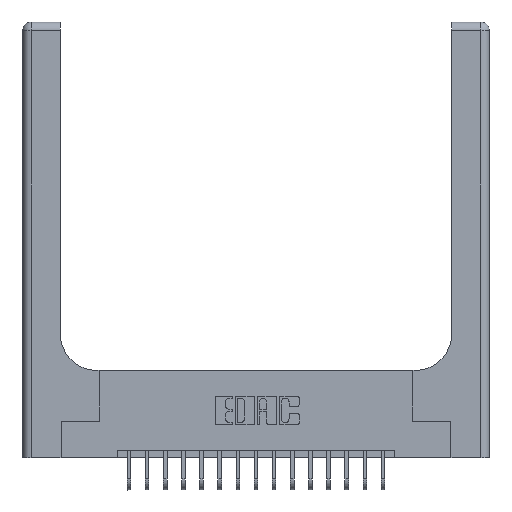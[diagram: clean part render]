
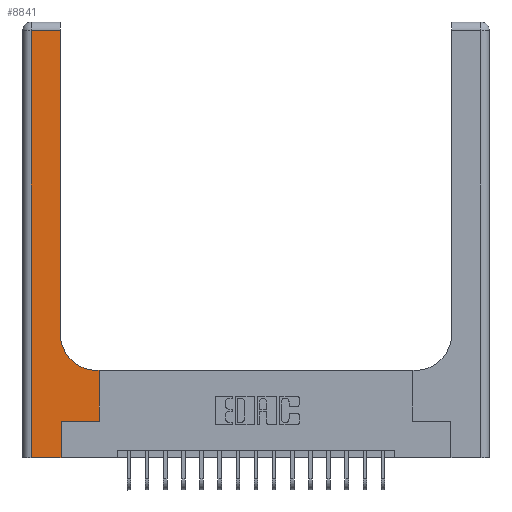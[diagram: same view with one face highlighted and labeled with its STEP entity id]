
A CAD part, top view. The second image highlights one B-rep face of the part: STEP entity #8841.
In plain terms, the highlighted planar face has unit normal (0, 0, 1).
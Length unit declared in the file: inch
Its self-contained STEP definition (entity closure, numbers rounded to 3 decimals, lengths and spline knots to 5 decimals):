
#110 = EDGE_CURVE ( 'NONE', #10247, #282, #4777, .T. ) ;
#227 = CARTESIAN_POINT ( 'NONE',  ( 0.26, 2.94, 0.37 ) ) ;
#282 = VERTEX_POINT ( 'NONE', #8827 ) ;
#332 = LINE ( 'NONE', #10651, #8175 ) ;
#1098 = VECTOR ( 'NONE', #10964, 39.37008 ) ;
#1131 = LINE ( 'NONE', #14423, #17380 ) ;
#1418 = DIRECTION ( 'NONE',  ( 0., 0., -1. ) ) ;
#1751 = DIRECTION ( 'NONE',  ( 0., 0., -1. ) ) ;
#2239 = DIRECTION ( 'NONE',  ( 0., 1., 0. ) ) ;
#2355 = LINE ( 'NONE', #10632, #17366 ) ;
#2410 = EDGE_CURVE ( 'NONE', #8471, #15333, #11930, .T. ) ;
#3221 = EDGE_CURVE ( 'NONE', #282, #6428, #16419, .T. ) ;
#3464 = DIRECTION ( 'NONE',  ( 0., 1., 0. ) ) ;
#3870 = EDGE_CURVE ( 'NONE', #9569, #4636, #1131, .T. ) ;
#4448 = EDGE_LOOP ( 'NONE', ( #10275, #13189, #12014, #18849, #20106, #5891, #11778, #18100, #5657 ) ) ;
#4636 = VERTEX_POINT ( 'NONE', #15033 ) ;
#4660 = CARTESIAN_POINT ( 'NONE',  ( 0., 2.94, 0.37 ) ) ;
#4743 = DIRECTION ( 'NONE',  ( 0., 1., 0. ) ) ;
#4777 = LINE ( 'NONE', #7968, #1098 ) ;
#4818 = VERTEX_POINT ( 'NONE', #17353 ) ;
#5657 = ORIENTED_EDGE ( 'NONE', *, *, #3221, .T. ) ;
#5891 = ORIENTED_EDGE ( 'NONE', *, *, #7492, .T. ) ;
#6418 = CARTESIAN_POINT ( 'NONE',  ( 0.265, 0., 0.37 ) ) ;
#6428 = VERTEX_POINT ( 'NONE', #19565 ) ;
#6442 = EDGE_CURVE ( 'NONE', #14029, #10247, #332, .T. ) ;
#6672 = VECTOR ( 'NONE', #13729, 39.37008 ) ;
#7492 = EDGE_CURVE ( 'NONE', #4636, #14029, #11863, .T. ) ;
#7692 = VECTOR ( 'NONE', #4743, 39.37008 ) ;
#7725 = CARTESIAN_POINT ( 'NONE',  ( 0.51, 0.85, 0.37 ) ) ;
#7849 = DIRECTION ( 'NONE',  ( 1., 0., 0. ) ) ;
#7946 = VECTOR ( 'NONE', #12591, 39.37008 ) ;
#7968 = CARTESIAN_POINT ( 'NONE',  ( 0.26, 0.6, 0.37 ) ) ;
#7972 = CARTESIAN_POINT ( 'NONE',  ( 0.528, 0.6, 0.37 ) ) ;
#8175 = VECTOR ( 'NONE', #2239, 39.37008 ) ;
#8471 = VERTEX_POINT ( 'NONE', #227 ) ;
#8827 = CARTESIAN_POINT ( 'NONE',  ( 0.51, 0.6, 0.37 ) ) ;
#8841 = ADVANCED_FACE ( 'NONE', ( #13992 ), #14141, .F. ) ;
#9569 = VERTEX_POINT ( 'NONE', #6418 ) ;
#9953 = DIRECTION ( 'NONE',  ( -1., 0., 0. ) ) ;
#10247 = VERTEX_POINT ( 'NONE', #7972 ) ;
#10275 = ORIENTED_EDGE ( 'NONE', *, *, #15629, .T. ) ;
#10495 = CARTESIAN_POINT ( 'NONE',  ( 0., 0., 0.37 ) ) ;
#10632 = CARTESIAN_POINT ( 'NONE',  ( 0.06, 3., 0.37 ) ) ;
#10651 = CARTESIAN_POINT ( 'NONE',  ( 0.528, 0.25, 0.37 ) ) ;
#10964 = DIRECTION ( 'NONE',  ( -1., 0., 0. ) ) ;
#11034 = CARTESIAN_POINT ( 'NONE',  ( 0.26, 3., 0.37 ) ) ;
#11778 = ORIENTED_EDGE ( 'NONE', *, *, #6442, .T. ) ;
#11863 = LINE ( 'NONE', #18374, #6672 ) ;
#11930 = LINE ( 'NONE', #4660, #7946 ) ;
#12014 = ORIENTED_EDGE ( 'NONE', *, *, #13231, .T. ) ;
#12591 = DIRECTION ( 'NONE',  ( -1., 0., 0. ) ) ;
#12728 = DIRECTION ( 'NONE',  ( 0., -1., 0. ) ) ;
#12943 = CARTESIAN_POINT ( 'NONE',  ( 0.528, 0.25, 0.37 ) ) ;
#13189 = ORIENTED_EDGE ( 'NONE', *, *, #2410, .T. ) ;
#13231 = EDGE_CURVE ( 'NONE', #15333, #4818, #2355, .T. ) ;
#13729 = DIRECTION ( 'NONE',  ( 1., 0., 0. ) ) ;
#13992 = FACE_OUTER_BOUND ( 'NONE', #4448, .T. ) ;
#14029 = VERTEX_POINT ( 'NONE', #12943 ) ;
#14070 = AXIS2_PLACEMENT_3D ( 'NONE', #7725, #1418, #7849 ) ;
#14141 = PLANE ( 'NONE',  #14687 ) ;
#14423 = CARTESIAN_POINT ( 'NONE',  ( 0.265, 0., 0.37 ) ) ;
#14687 = AXIS2_PLACEMENT_3D ( 'NONE', #17601, #1751, #9953 ) ;
#14967 = CARTESIAN_POINT ( 'NONE',  ( 0.06, 2.94, 0.37 ) ) ;
#15033 = CARTESIAN_POINT ( 'NONE',  ( 0.265, 0.25, 0.37 ) ) ;
#15333 = VERTEX_POINT ( 'NONE', #14967 ) ;
#15421 = DIRECTION ( 'NONE',  ( 1., 0., 0. ) ) ;
#15596 = LINE ( 'NONE', #11034, #7692 ) ;
#15629 = EDGE_CURVE ( 'NONE', #6428, #8471, #15596, .T. ) ;
#15730 = LINE ( 'NONE', #10495, #19957 ) ;
#16419 = CIRCLE ( 'NONE', #14070, 0.25 ) ;
#17353 = CARTESIAN_POINT ( 'NONE',  ( 0.06, 0., 0.37 ) ) ;
#17366 = VECTOR ( 'NONE', #12728, 39.37008 ) ;
#17380 = VECTOR ( 'NONE', #3464, 39.37008 ) ;
#17601 = CARTESIAN_POINT ( 'NONE',  ( 0., 3., 0.37 ) ) ;
#18100 = ORIENTED_EDGE ( 'NONE', *, *, #110, .T. ) ;
#18374 = CARTESIAN_POINT ( 'NONE',  ( 0.265, 0.25, 0.37 ) ) ;
#18849 = ORIENTED_EDGE ( 'NONE', *, *, #19763, .T. ) ;
#19565 = CARTESIAN_POINT ( 'NONE',  ( 0.26, 0.85, 0.37 ) ) ;
#19763 = EDGE_CURVE ( 'NONE', #4818, #9569, #15730, .T. ) ;
#19957 = VECTOR ( 'NONE', #15421, 39.37008 ) ;
#20106 = ORIENTED_EDGE ( 'NONE', *, *, #3870, .T. ) ;
